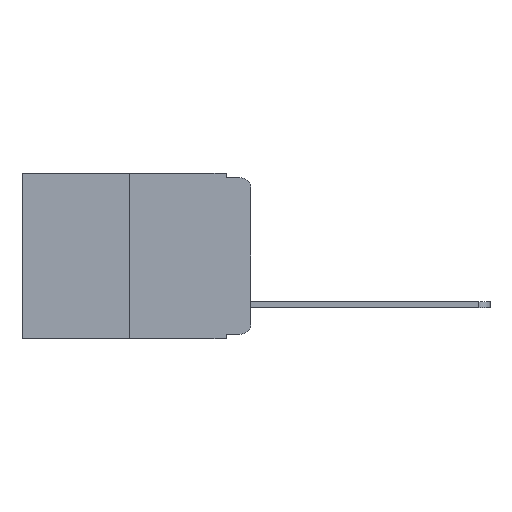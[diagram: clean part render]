
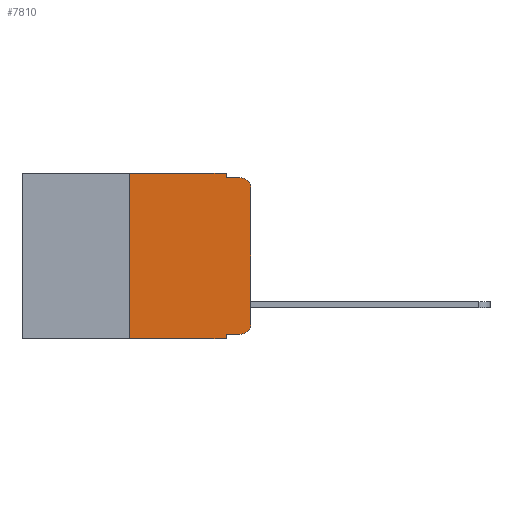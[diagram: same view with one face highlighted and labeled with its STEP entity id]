
A CAD part, left-side view. The second image highlights one B-rep face of the part: STEP entity #7810.
In plain terms, the highlighted planar face has unit normal (-1, 0, 0).
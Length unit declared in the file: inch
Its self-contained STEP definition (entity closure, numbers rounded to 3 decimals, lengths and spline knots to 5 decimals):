
#101 = ORIENTED_EDGE ( 'NONE', *, *, #16286, .T. ) ;
#588 = CARTESIAN_POINT ( 'NONE',  ( 0., 0.051, 0. ) ) ;
#594 = CARTESIAN_POINT ( 'NONE',  ( 0., 0.051, -0.01 ) ) ;
#667 = LINE ( 'NONE', #588, #13548 ) ;
#758 = CARTESIAN_POINT ( 'NONE',  ( 0., 0.02, -0.01 ) ) ;
#820 = EDGE_CURVE ( 'NONE', #12090, #18452, #7295, .T. ) ;
#1132 = VERTEX_POINT ( 'NONE', #13057 ) ;
#1236 = VERTEX_POINT ( 'NONE', #10118 ) ;
#1526 = DIRECTION ( 'NONE',  ( 0., 0., -1. ) ) ;
#1730 = EDGE_CURVE ( 'NONE', #18276, #12090, #20806, .T. ) ;
#1990 = DIRECTION ( 'NONE',  ( 0., 0., -1. ) ) ;
#2137 = DIRECTION ( 'NONE',  ( 0., 0., -1. ) ) ;
#2195 = CARTESIAN_POINT ( 'NONE',  ( 0., 0., 0. ) ) ;
#2480 = ORIENTED_EDGE ( 'NONE', *, *, #8415, .T. ) ;
#2741 = VECTOR ( 'NONE', #9226, 39.37008 ) ;
#3159 = ORIENTED_EDGE ( 'NONE', *, *, #14535, .T. ) ;
#3589 = VECTOR ( 'NONE', #12745, 39.37008 ) ;
#4024 = VECTOR ( 'NONE', #19739, 39.37008 ) ;
#4281 = CARTESIAN_POINT ( 'NONE',  ( 0., 0.051, -0.01 ) ) ;
#4349 = CARTESIAN_POINT ( 'NONE',  ( 0., 0.051, -0.333 ) ) ;
#5395 = EDGE_CURVE ( 'NONE', #18452, #13444, #15396, .T. ) ;
#5564 = AXIS2_PLACEMENT_3D ( 'NONE', #16885, #12053, #1990 ) ;
#5653 = CARTESIAN_POINT ( 'NONE',  ( 0., 0.473, 0. ) ) ;
#6538 = LINE ( 'NONE', #594, #19372 ) ;
#6579 = DIRECTION ( 'NONE',  ( -1., 0., 0. ) ) ;
#6793 = DIRECTION ( 'NONE',  ( 0., 0., -1. ) ) ;
#6875 = ORIENTED_EDGE ( 'NONE', *, *, #15709, .T. ) ;
#7039 = AXIS2_PLACEMENT_3D ( 'NONE', #21413, #6579, #1526 ) ;
#7295 = LINE ( 'NONE', #5653, #14374 ) ;
#7526 = ORIENTED_EDGE ( 'NONE', *, *, #14099, .F. ) ;
#7810 = ADVANCED_FACE ( 'NONE', ( #20185 ), #11801, .F. ) ;
#8415 = EDGE_CURVE ( 'NONE', #1236, #1132, #21434, .T. ) ;
#8512 = EDGE_CURVE ( 'NONE', #16971, #9010, #667, .T. ) ;
#8585 = CARTESIAN_POINT ( 'NONE',  ( 0., 0., -0.03 ) ) ;
#9010 = VERTEX_POINT ( 'NONE', #18401 ) ;
#9139 = VERTEX_POINT ( 'NONE', #8585 ) ;
#9226 = DIRECTION ( 'NONE',  ( 0., -1., 0. ) ) ;
#9275 = CARTESIAN_POINT ( 'NONE',  ( 0., 0.25, -0.343 ) ) ;
#9807 = CARTESIAN_POINT ( 'NONE',  ( 0., 0.051, 0. ) ) ;
#10118 = CARTESIAN_POINT ( 'NONE',  ( 0., 0.02, -0.333 ) ) ;
#10168 = VECTOR ( 'NONE', #2137, 39.37008 ) ;
#10376 = ORIENTED_EDGE ( 'NONE', *, *, #5395, .F. ) ;
#10440 = EDGE_LOOP ( 'NONE', ( #6875, #16316, #7526, #10376, #20885, #14513, #3159, #14425, #101, #2480 ) ) ;
#10456 = DIRECTION ( 'NONE',  ( 0., -1., 0. ) ) ;
#11124 = CARTESIAN_POINT ( 'NONE',  ( 0., 0.051, -0.333 ) ) ;
#11704 = LINE ( 'NONE', #11124, #2741 ) ;
#11801 = PLANE ( 'NONE',  #15810 ) ;
#12039 = CIRCLE ( 'NONE', #7039, 0.02 ) ;
#12053 = DIRECTION ( 'NONE',  ( -1., 0., 0. ) ) ;
#12090 = VERTEX_POINT ( 'NONE', #20468 ) ;
#12549 = VECTOR ( 'NONE', #10456, 39.37008 ) ;
#12745 = DIRECTION ( 'NONE',  ( 0., 0., 1. ) ) ;
#13022 = CARTESIAN_POINT ( 'NONE',  ( 0., 0.473, -0.343 ) ) ;
#13057 = CARTESIAN_POINT ( 'NONE',  ( 0., 0., -0.313 ) ) ;
#13112 = EDGE_CURVE ( 'NONE', #9139, #18297, #12039, .T. ) ;
#13444 = VERTEX_POINT ( 'NONE', #4281 ) ;
#13548 = VECTOR ( 'NONE', #18979, 39.37008 ) ;
#14099 = EDGE_CURVE ( 'NONE', #13444, #18297, #6538, .T. ) ;
#14374 = VECTOR ( 'NONE', #17158, 39.37008 ) ;
#14425 = ORIENTED_EDGE ( 'NONE', *, *, #8512, .F. ) ;
#14513 = ORIENTED_EDGE ( 'NONE', *, *, #1730, .F. ) ;
#14535 = EDGE_CURVE ( 'NONE', #18276, #9010, #17022, .T. ) ;
#15396 = LINE ( 'NONE', #15840, #10168 ) ;
#15709 = EDGE_CURVE ( 'NONE', #1132, #9139, #16962, .T. ) ;
#15810 = AXIS2_PLACEMENT_3D ( 'NONE', #18722, #16777, #6793 ) ;
#15840 = CARTESIAN_POINT ( 'NONE',  ( 0., 0.051, 0. ) ) ;
#16286 = EDGE_CURVE ( 'NONE', #16971, #1236, #11704, .T. ) ;
#16316 = ORIENTED_EDGE ( 'NONE', *, *, #13112, .T. ) ;
#16777 = DIRECTION ( 'NONE',  ( 1., 0., 0. ) ) ;
#16885 = CARTESIAN_POINT ( 'NONE',  ( 0., 0.02, -0.313 ) ) ;
#16962 = LINE ( 'NONE', #2195, #3589 ) ;
#16971 = VERTEX_POINT ( 'NONE', #4349 ) ;
#17022 = LINE ( 'NONE', #13022, #12549 ) ;
#17158 = DIRECTION ( 'NONE',  ( 0., -1., 0. ) ) ;
#18078 = CARTESIAN_POINT ( 'NONE',  ( 0., 0.25, 0. ) ) ;
#18276 = VERTEX_POINT ( 'NONE', #9275 ) ;
#18297 = VERTEX_POINT ( 'NONE', #758 ) ;
#18401 = CARTESIAN_POINT ( 'NONE',  ( 0., 0.051, -0.343 ) ) ;
#18452 = VERTEX_POINT ( 'NONE', #9807 ) ;
#18722 = CARTESIAN_POINT ( 'NONE',  ( 0., 0.473, 0. ) ) ;
#18979 = DIRECTION ( 'NONE',  ( 0., 0., -1. ) ) ;
#18989 = DIRECTION ( 'NONE',  ( 0., -1., 0. ) ) ;
#19372 = VECTOR ( 'NONE', #18989, 39.37008 ) ;
#19739 = DIRECTION ( 'NONE',  ( 0., 0., 1. ) ) ;
#20185 = FACE_OUTER_BOUND ( 'NONE', #10440, .T. ) ;
#20468 = CARTESIAN_POINT ( 'NONE',  ( 0., 0.25, 0. ) ) ;
#20806 = LINE ( 'NONE', #18078, #4024 ) ;
#20885 = ORIENTED_EDGE ( 'NONE', *, *, #820, .F. ) ;
#21413 = CARTESIAN_POINT ( 'NONE',  ( 0., 0.02, -0.03 ) ) ;
#21434 = CIRCLE ( 'NONE', #5564, 0.02 ) ;
